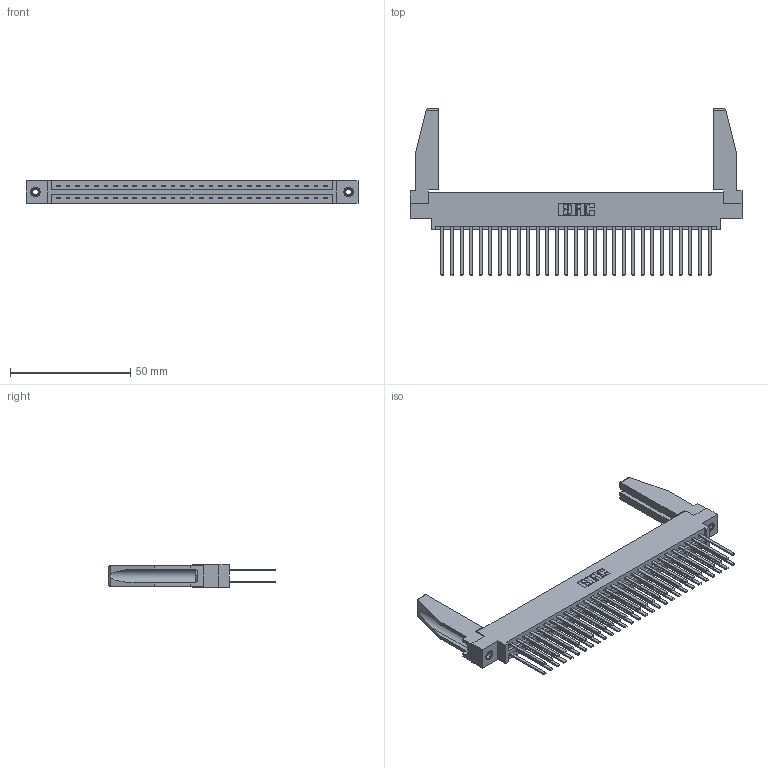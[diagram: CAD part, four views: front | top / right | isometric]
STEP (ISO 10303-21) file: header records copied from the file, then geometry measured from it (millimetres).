
FILE_DESCRIPTION (( 'STEP AP203' ), '1' );
FILE_NAME ('387-058-544-878.STEP', '2019-10-19T09:41:54', ( '' ), ( '' ), 'SwSTEP 2.0', 'SolidWorks 2016', '' );
FILE_SCHEMA (( 'CONFIG_CONTROL_DESIGN' ));
Length unit declared in the file: inch
Products named in the file (5): 337 Part_0.170 Offset - 0.156 Dia-TI; 345-292-001_345-293-144; 307-220-078; 387-058-544-878; 345-250-001_345-250-001-102
Assembly tree (63 placements, depth 2):
  387-058-544-878
    337 Part_0.170 Offset - 0.156 Dia-TI
    345-292-001_345-293-144  x58
    345-250-001_345-250-001-102  x2
    307-220-078  x2
Bounding box: 137.92 x 69.09 x 9.4 mm (x, y, z)
Volume: 19051.1 mm3; surface area: 23490.9 mm2
Topology: 63 solids, 63 shells, 3032 faces, 8947 edges, 5878 vertices
Faces by surface type: plane 2130, cylinder 886, cone 12, torus 4
Entity records: 26554 total; most frequent: CARTESIAN_POINT 4484, ORIENTED_EDGE 4376, DIRECTION 3840, EDGE_CURVE 2188, VECTOR 2026, LINE 2026, VERTEX_POINT 1452, AXIS2_PLACEMENT_3D 907
